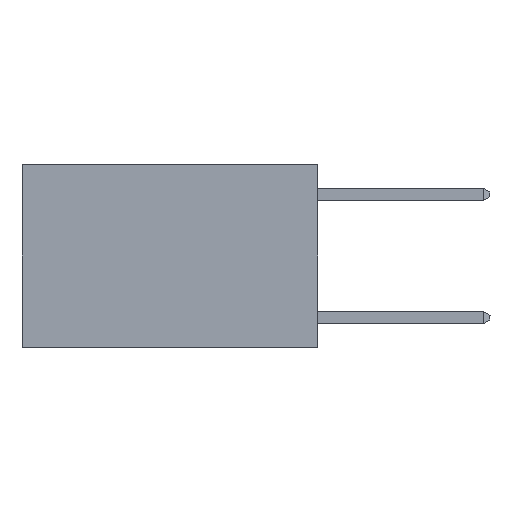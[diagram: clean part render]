
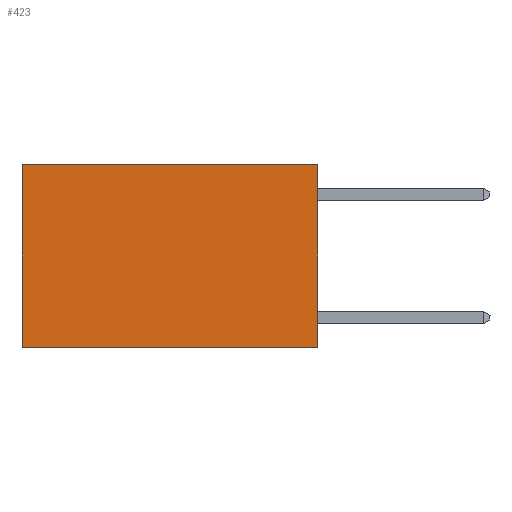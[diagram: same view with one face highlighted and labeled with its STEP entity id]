
A CAD part, left-side view. The second image highlights one B-rep face of the part: STEP entity #423.
In plain terms, the highlighted planar face has unit normal (-1, 0, 0).
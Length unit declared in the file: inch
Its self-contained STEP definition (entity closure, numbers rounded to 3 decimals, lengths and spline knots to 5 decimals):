
#32 = LINE ( 'NONE', #10556, #8242 ) ;
#423 = ADVANCED_FACE ( 'NONE', ( #8349 ), #8535, .F. ) ;
#589 = DIRECTION ( 'NONE',  ( 0., 1., 0. ) ) ;
#828 = CARTESIAN_POINT ( 'NONE',  ( 0.2625, 0.6, -0.37 ) ) ;
#907 = CARTESIAN_POINT ( 'NONE',  ( 0.2625, 0., 0. ) ) ;
#1134 = ORIENTED_EDGE ( 'NONE', *, *, #5043, .T. ) ;
#1809 = LINE ( 'NONE', #5899, #12600 ) ;
#2003 = DIRECTION ( 'NONE',  ( 0., 0., -1. ) ) ;
#2732 = ORIENTED_EDGE ( 'NONE', *, *, #11695, .F. ) ;
#3464 = DIRECTION ( 'NONE',  ( 0., 0., -1. ) ) ;
#3567 = EDGE_CURVE ( 'NONE', #4346, #11235, #10147, .T. ) ;
#3742 = EDGE_CURVE ( 'NONE', #5535, #7825, #32, .T. ) ;
#3954 = VECTOR ( 'NONE', #589, 39.37008 ) ;
#4110 = DIRECTION ( 'NONE',  ( 1., 0., 0. ) ) ;
#4165 = CARTESIAN_POINT ( 'NONE',  ( 0.2625, 0., -0.37 ) ) ;
#4346 = VERTEX_POINT ( 'NONE', #11414 ) ;
#5043 = EDGE_CURVE ( 'NONE', #4346, #5535, #9337, .T. ) ;
#5050 = ORIENTED_EDGE ( 'NONE', *, *, #3742, .T. ) ;
#5094 = VECTOR ( 'NONE', #7070, 39.37008 ) ;
#5177 = AXIS2_PLACEMENT_3D ( 'NONE', #12700, #4110, #2003 ) ;
#5535 = VERTEX_POINT ( 'NONE', #9497 ) ;
#5899 = CARTESIAN_POINT ( 'NONE',  ( 0.2625, 0., -0.37 ) ) ;
#7070 = DIRECTION ( 'NONE',  ( 0., 0., -1. ) ) ;
#7661 = EDGE_LOOP ( 'NONE', ( #5050, #2732, #9595, #1134 ) ) ;
#7767 = CARTESIAN_POINT ( 'NONE',  ( 0.2625, 0., 0. ) ) ;
#7825 = VERTEX_POINT ( 'NONE', #828 ) ;
#8242 = VECTOR ( 'NONE', #3464, 39.37008 ) ;
#8349 = FACE_OUTER_BOUND ( 'NONE', #7661, .T. ) ;
#8535 = PLANE ( 'NONE',  #5177 ) ;
#9337 = LINE ( 'NONE', #7767, #3954 ) ;
#9497 = CARTESIAN_POINT ( 'NONE',  ( 0.2625, 0.6, 0. ) ) ;
#9595 = ORIENTED_EDGE ( 'NONE', *, *, #3567, .F. ) ;
#10147 = LINE ( 'NONE', #907, #5094 ) ;
#10556 = CARTESIAN_POINT ( 'NONE',  ( 0.2625, 0.6, 0. ) ) ;
#11235 = VERTEX_POINT ( 'NONE', #4165 ) ;
#11414 = CARTESIAN_POINT ( 'NONE',  ( 0.2625, 0., 0. ) ) ;
#11695 = EDGE_CURVE ( 'NONE', #11235, #7825, #1809, .T. ) ;
#11925 = DIRECTION ( 'NONE',  ( 0., 1., 0. ) ) ;
#12600 = VECTOR ( 'NONE', #11925, 39.37008 ) ;
#12700 = CARTESIAN_POINT ( 'NONE',  ( 0.2625, 0., 0. ) ) ;
